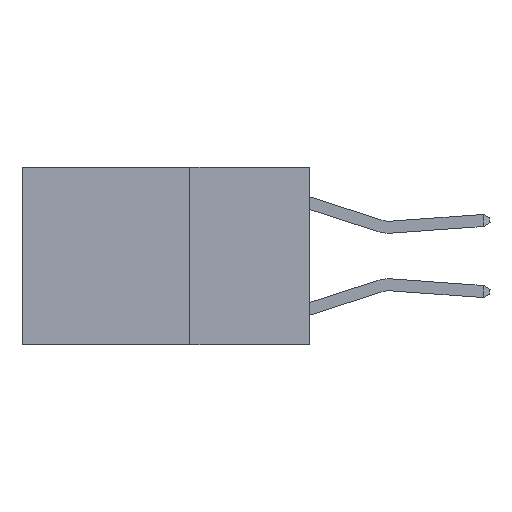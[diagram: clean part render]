
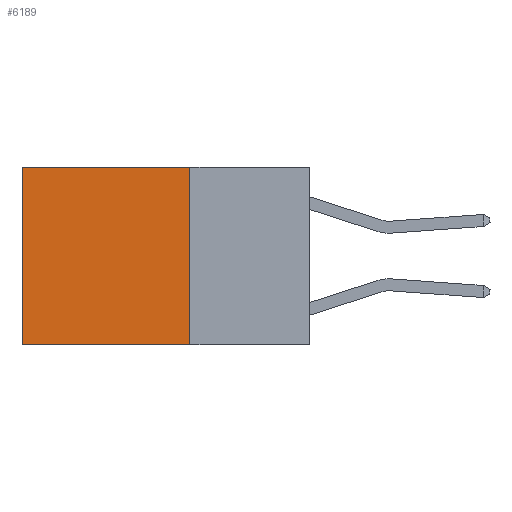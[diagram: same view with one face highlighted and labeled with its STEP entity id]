
A CAD part, left-side view. The second image highlights one B-rep face of the part: STEP entity #6189.
In plain terms, the highlighted planar face has unit normal (-1, 0, 0).
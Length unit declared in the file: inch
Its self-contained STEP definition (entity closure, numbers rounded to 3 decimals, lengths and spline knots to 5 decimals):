
#323 = ORIENTED_EDGE ( 'NONE', *, *, #10544, .T. ) ;
#1205 = ORIENTED_EDGE ( 'NONE', *, *, #8240, .F. ) ;
#1298 = VERTEX_POINT ( 'NONE', #9478 ) ;
#1827 = CARTESIAN_POINT ( 'NONE',  ( 0.2625, 0.25, 0. ) ) ;
#2792 = VERTEX_POINT ( 'NONE', #5939 ) ;
#3326 = LINE ( 'NONE', #9983, #6860 ) ;
#3364 = VECTOR ( 'NONE', #9220, 39.37008 ) ;
#3519 = DIRECTION ( 'NONE',  ( 0., 0., -1. ) ) ;
#4260 = CARTESIAN_POINT ( 'NONE',  ( 0.2625, 0.25, -0.37 ) ) ;
#4332 = FACE_OUTER_BOUND ( 'NONE', #8768, .T. ) ;
#4676 = EDGE_CURVE ( 'NONE', #10719, #2792, #6571, .T. ) ;
#4702 = LINE ( 'NONE', #6314, #6741 ) ;
#5798 = DIRECTION ( 'NONE',  ( 0., 0., -1. ) ) ;
#5939 = CARTESIAN_POINT ( 'NONE',  ( 0.2625, 0.6, -0.37 ) ) ;
#6092 = EDGE_CURVE ( 'NONE', #6260, #1298, #3326, .T. ) ;
#6189 = ADVANCED_FACE ( 'NONE', ( #4332 ), #9262, .F. ) ;
#6260 = VERTEX_POINT ( 'NONE', #7903 ) ;
#6314 = CARTESIAN_POINT ( 'NONE',  ( 0.2625, 0.25, 0. ) ) ;
#6571 = LINE ( 'NONE', #8244, #8788 ) ;
#6585 = DIRECTION ( 'NONE',  ( 1., 0., 0. ) ) ;
#6698 = CARTESIAN_POINT ( 'NONE',  ( 0.2625, 0.6, 0. ) ) ;
#6741 = VECTOR ( 'NONE', #8824, 39.37008 ) ;
#6860 = VECTOR ( 'NONE', #3519, 39.37008 ) ;
#7903 = CARTESIAN_POINT ( 'NONE',  ( 0.2625, 0.25, 0. ) ) ;
#8141 = AXIS2_PLACEMENT_3D ( 'NONE', #1827, #6585, #8372 ) ;
#8240 = EDGE_CURVE ( 'NONE', #1298, #2792, #10933, .T. ) ;
#8244 = CARTESIAN_POINT ( 'NONE',  ( 0.2625, 0.6, 0. ) ) ;
#8372 = DIRECTION ( 'NONE',  ( 0., 0., -1. ) ) ;
#8768 = EDGE_LOOP ( 'NONE', ( #10062, #1205, #9227, #323 ) ) ;
#8788 = VECTOR ( 'NONE', #5798, 39.37008 ) ;
#8824 = DIRECTION ( 'NONE',  ( 0., 1., 0. ) ) ;
#9220 = DIRECTION ( 'NONE',  ( 0., 1., 0. ) ) ;
#9227 = ORIENTED_EDGE ( 'NONE', *, *, #6092, .F. ) ;
#9262 = PLANE ( 'NONE',  #8141 ) ;
#9478 = CARTESIAN_POINT ( 'NONE',  ( 0.2625, 0.25, -0.37 ) ) ;
#9983 = CARTESIAN_POINT ( 'NONE',  ( 0.2625, 0.25, 0. ) ) ;
#10062 = ORIENTED_EDGE ( 'NONE', *, *, #4676, .T. ) ;
#10544 = EDGE_CURVE ( 'NONE', #6260, #10719, #4702, .T. ) ;
#10719 = VERTEX_POINT ( 'NONE', #6698 ) ;
#10933 = LINE ( 'NONE', #4260, #3364 ) ;
